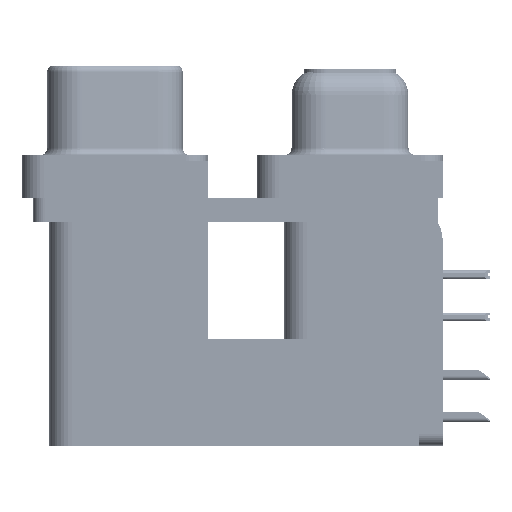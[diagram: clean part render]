
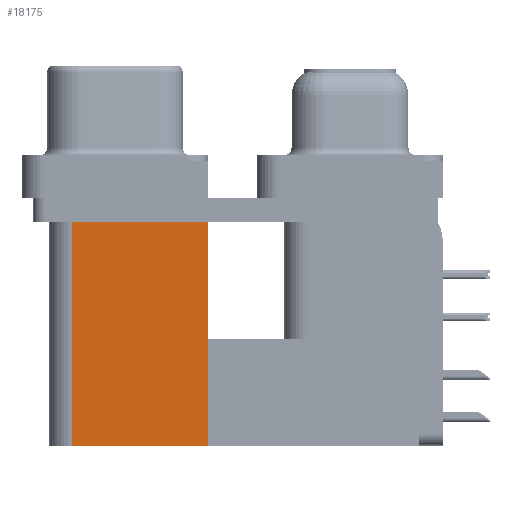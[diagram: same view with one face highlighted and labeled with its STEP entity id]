
A CAD part, left-side view. The second image highlights one B-rep face of the part: STEP entity #18175.
In plain terms, the highlighted planar face has unit normal (-1, 0, 0).
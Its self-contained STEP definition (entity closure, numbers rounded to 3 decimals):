
#2689 = PLANE ( 'NONE',  #51397 ) ;
#5253 = CARTESIAN_POINT ( 'NONE',  ( 3.79, 9.6, -19.2 ) ) ;
#5867 = CARTESIAN_POINT ( 'NONE',  ( 3.79, 18.8, -19.2 ) ) ;
#6087 = VECTOR ( 'NONE', #15806, 1000. ) ;
#6962 = EDGE_CURVE ( 'NONE', #36544, #60163, #30998, .T. ) ;
#9808 = DIRECTION ( 'NONE',  ( 0., 0., 1. ) ) ;
#11974 = ORIENTED_EDGE ( 'NONE', *, *, #49451, .T. ) ;
#13810 = ORIENTED_EDGE ( 'NONE', *, *, #6962, .T. ) ;
#15606 = EDGE_LOOP ( 'NONE', ( #11974, #63438, #17389, #13810 ) ) ;
#15806 = DIRECTION ( 'NONE',  ( 0., 0., 1. ) ) ;
#17389 = ORIENTED_EDGE ( 'NONE', *, *, #55077, .F. ) ;
#18087 = CARTESIAN_POINT ( 'NONE',  ( 3.79, 9.6, -19.2 ) ) ;
#18175 = ADVANCED_FACE ( 'NONE', ( #58157 ), #2689, .F. ) ;
#22007 = DIRECTION ( 'NONE',  ( 0., 1., 0. ) ) ;
#24623 = EDGE_CURVE ( 'NONE', #67285, #66138, #30867, .T. ) ;
#24730 = CARTESIAN_POINT ( 'NONE',  ( 3.79, 18.8, -2.5 ) ) ;
#30867 = LINE ( 'NONE', #5867, #6087 ) ;
#30998 = LINE ( 'NONE', #56689, #53408 ) ;
#36544 = VERTEX_POINT ( 'NONE', #5253 ) ;
#41962 = DIRECTION ( 'NONE',  ( 0., 1., 0. ) ) ;
#42544 = LINE ( 'NONE', #48695, #48356 ) ;
#47102 = LINE ( 'NONE', #52920, #47354 ) ;
#47354 = VECTOR ( 'NONE', #41962, 1000. ) ;
#48356 = VECTOR ( 'NONE', #22007, 1000. ) ;
#48695 = CARTESIAN_POINT ( 'NONE',  ( 3.79, 9.6, -19.2 ) ) ;
#49451 = EDGE_CURVE ( 'NONE', #60163, #66138, #47102, .T. ) ;
#51397 = AXIS2_PLACEMENT_3D ( 'NONE', #18087, #59184, #54050 ) ;
#52920 = CARTESIAN_POINT ( 'NONE',  ( 3.79, 9.6, -2.5 ) ) ;
#53196 = CARTESIAN_POINT ( 'NONE',  ( 3.79, 18.8, -19.2 ) ) ;
#53408 = VECTOR ( 'NONE', #9808, 1000. ) ;
#54050 = DIRECTION ( 'NONE',  ( 0., 0., -1. ) ) ;
#55077 = EDGE_CURVE ( 'NONE', #36544, #67285, #42544, .T. ) ;
#56689 = CARTESIAN_POINT ( 'NONE',  ( 3.79, 9.6, -19.2 ) ) ;
#57052 = CARTESIAN_POINT ( 'NONE',  ( 3.79, 9.6, -2.5 ) ) ;
#58157 = FACE_OUTER_BOUND ( 'NONE', #15606, .T. ) ;
#59184 = DIRECTION ( 'NONE',  ( 1., 0., 0. ) ) ;
#60163 = VERTEX_POINT ( 'NONE', #57052 ) ;
#63438 = ORIENTED_EDGE ( 'NONE', *, *, #24623, .F. ) ;
#66138 = VERTEX_POINT ( 'NONE', #24730 ) ;
#67285 = VERTEX_POINT ( 'NONE', #53196 ) ;
